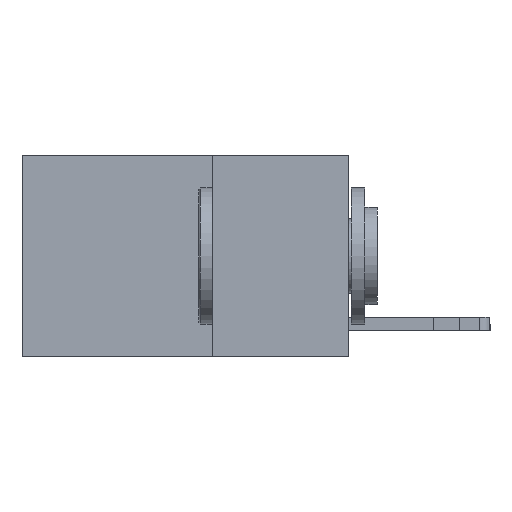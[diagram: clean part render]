
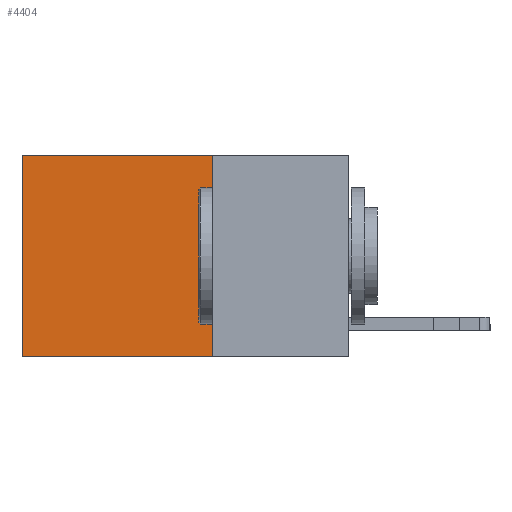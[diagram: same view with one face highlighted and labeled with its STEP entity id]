
A CAD part, left-side view. The second image highlights one B-rep face of the part: STEP entity #4404.
In plain terms, the highlighted planar face has unit normal (-1, 0, 0).
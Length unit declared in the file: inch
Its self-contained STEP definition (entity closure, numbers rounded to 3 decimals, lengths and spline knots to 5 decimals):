
#254 = LINE ( 'NONE', #3250, #10553 ) ;
#1818 = DIRECTION ( 'NONE',  ( 1., 0., 0. ) ) ;
#2052 = ORIENTED_EDGE ( 'NONE', *, *, #5529, .F. ) ;
#3238 = EDGE_LOOP ( 'NONE', ( #7886, #2052, #9294, #17395 ) ) ;
#3250 = CARTESIAN_POINT ( 'NONE',  ( 0.2625, 0.25, 0. ) ) ;
#3826 = LINE ( 'NONE', #5252, #5651 ) ;
#4034 = VERTEX_POINT ( 'NONE', #7917 ) ;
#4404 = ADVANCED_FACE ( 'NONE', ( #6755 ), #10978, .F. ) ;
#4575 = LINE ( 'NONE', #15476, #7737 ) ;
#4622 = VECTOR ( 'NONE', #20345, 39.37008 ) ;
#4908 = DIRECTION ( 'NONE',  ( 0., 0., -1. ) ) ;
#5146 = VERTEX_POINT ( 'NONE', #18949 ) ;
#5252 = CARTESIAN_POINT ( 'NONE',  ( 0.2625, 0.6, 0. ) ) ;
#5529 = EDGE_CURVE ( 'NONE', #5146, #12434, #5846, .T. ) ;
#5651 = VECTOR ( 'NONE', #8140, 39.37008 ) ;
#5846 = LINE ( 'NONE', #10670, #4622 ) ;
#6755 = FACE_OUTER_BOUND ( 'NONE', #3238, .T. ) ;
#6783 = EDGE_CURVE ( 'NONE', #4034, #13824, #254, .T. ) ;
#7730 = CARTESIAN_POINT ( 'NONE',  ( 0.2625, 0.6, 0. ) ) ;
#7737 = VECTOR ( 'NONE', #7850, 39.37008 ) ;
#7850 = DIRECTION ( 'NONE',  ( 0., 0., -1. ) ) ;
#7886 = ORIENTED_EDGE ( 'NONE', *, *, #18290, .T. ) ;
#7917 = CARTESIAN_POINT ( 'NONE',  ( 0.2625, 0.25, 0. ) ) ;
#8140 = DIRECTION ( 'NONE',  ( 0., 0., -1. ) ) ;
#9294 = ORIENTED_EDGE ( 'NONE', *, *, #12305, .F. ) ;
#10553 = VECTOR ( 'NONE', #12506, 39.37008 ) ;
#10670 = CARTESIAN_POINT ( 'NONE',  ( 0.2625, 0.25, -0.37 ) ) ;
#10978 = PLANE ( 'NONE',  #18785 ) ;
#12305 = EDGE_CURVE ( 'NONE', #4034, #5146, #4575, .T. ) ;
#12434 = VERTEX_POINT ( 'NONE', #19069 ) ;
#12506 = DIRECTION ( 'NONE',  ( 0., 1., 0. ) ) ;
#13824 = VERTEX_POINT ( 'NONE', #7730 ) ;
#14581 = CARTESIAN_POINT ( 'NONE',  ( 0.2625, 0.25, 0. ) ) ;
#15476 = CARTESIAN_POINT ( 'NONE',  ( 0.2625, 0.25, 0. ) ) ;
#17395 = ORIENTED_EDGE ( 'NONE', *, *, #6783, .T. ) ;
#18290 = EDGE_CURVE ( 'NONE', #13824, #12434, #3826, .T. ) ;
#18785 = AXIS2_PLACEMENT_3D ( 'NONE', #14581, #1818, #4908 ) ;
#18949 = CARTESIAN_POINT ( 'NONE',  ( 0.2625, 0.25, -0.37 ) ) ;
#19069 = CARTESIAN_POINT ( 'NONE',  ( 0.2625, 0.6, -0.37 ) ) ;
#20345 = DIRECTION ( 'NONE',  ( 0., 1., 0. ) ) ;
